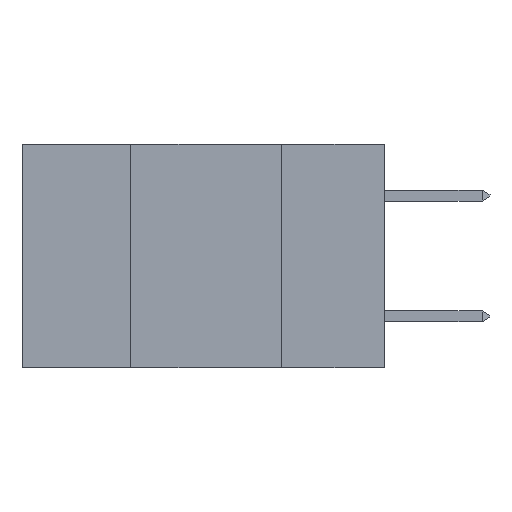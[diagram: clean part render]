
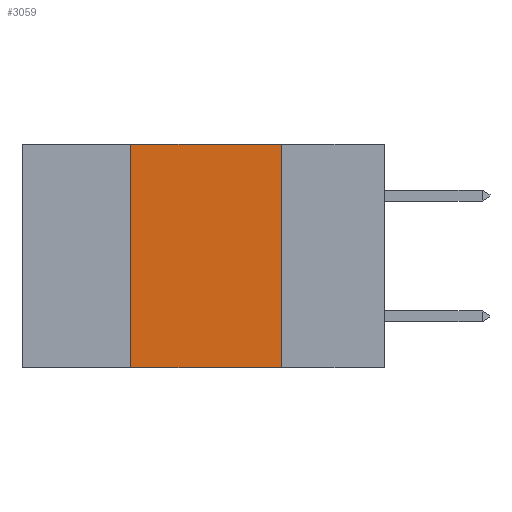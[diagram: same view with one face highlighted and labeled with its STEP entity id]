
A CAD part, left-side view. The second image highlights one B-rep face of the part: STEP entity #3059.
In plain terms, the highlighted planar face has unit normal (-1, 0, 0).
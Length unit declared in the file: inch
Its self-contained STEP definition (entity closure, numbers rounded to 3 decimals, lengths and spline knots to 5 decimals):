
#133 = VECTOR ( 'NONE', #5936, 39.37008 ) ;
#2025 = CARTESIAN_POINT ( 'NONE',  ( 0., 0.17, 0. ) ) ;
#3059 = ADVANCED_FACE ( 'NONE', ( #3275 ), #4996, .F. ) ;
#3275 = FACE_OUTER_BOUND ( 'NONE', #11206, .T. ) ;
#3481 = DIRECTION ( 'NONE',  ( 1., 0., 0. ) ) ;
#4345 = CARTESIAN_POINT ( 'NONE',  ( 0., 0.42, 0. ) ) ;
#4996 = PLANE ( 'NONE',  #13229 ) ;
#5587 = EDGE_CURVE ( 'NONE', #12993, #18678, #8573, .T. ) ;
#5814 = VERTEX_POINT ( 'NONE', #18926 ) ;
#5936 = DIRECTION ( 'NONE',  ( 0., 0., 1. ) ) ;
#6013 = ORIENTED_EDGE ( 'NONE', *, *, #13463, .F. ) ;
#7469 = ORIENTED_EDGE ( 'NONE', *, *, #20744, .F. ) ;
#7854 = ORIENTED_EDGE ( 'NONE', *, *, #13422, .F. ) ;
#8573 = LINE ( 'NONE', #15382, #11832 ) ;
#9318 = VERTEX_POINT ( 'NONE', #20121 ) ;
#9936 = CARTESIAN_POINT ( 'NONE',  ( 0., 0.6, 0. ) ) ;
#11185 = LINE ( 'NONE', #12137, #12690 ) ;
#11206 = EDGE_LOOP ( 'NONE', ( #7469, #7854, #6013, #16573 ) ) ;
#11832 = VECTOR ( 'NONE', #15319, 39.37008 ) ;
#11939 = LINE ( 'NONE', #4345, #133 ) ;
#12137 = CARTESIAN_POINT ( 'NONE',  ( 0., 0.6, 0. ) ) ;
#12690 = VECTOR ( 'NONE', #12712, 39.37008 ) ;
#12712 = DIRECTION ( 'NONE',  ( 0., -1., 0. ) ) ;
#12993 = VERTEX_POINT ( 'NONE', #19839 ) ;
#13229 = AXIS2_PLACEMENT_3D ( 'NONE', #9936, #3481, #16271 ) ;
#13422 = EDGE_CURVE ( 'NONE', #9318, #5814, #11185, .T. ) ;
#13463 = EDGE_CURVE ( 'NONE', #12993, #9318, #11939, .T. ) ;
#13984 = LINE ( 'NONE', #2025, #14480 ) ;
#14480 = VECTOR ( 'NONE', #19809, 39.37008 ) ;
#15319 = DIRECTION ( 'NONE',  ( 0., -1., 0. ) ) ;
#15382 = CARTESIAN_POINT ( 'NONE',  ( 0., 0.6, -0.37 ) ) ;
#16271 = DIRECTION ( 'NONE',  ( 0., 0., -1. ) ) ;
#16573 = ORIENTED_EDGE ( 'NONE', *, *, #5587, .T. ) ;
#18247 = CARTESIAN_POINT ( 'NONE',  ( 0., 0.17, -0.37 ) ) ;
#18678 = VERTEX_POINT ( 'NONE', #18247 ) ;
#18926 = CARTESIAN_POINT ( 'NONE',  ( 0., 0.17, 0. ) ) ;
#19809 = DIRECTION ( 'NONE',  ( 0., 0., -1. ) ) ;
#19839 = CARTESIAN_POINT ( 'NONE',  ( 0., 0.42, -0.37 ) ) ;
#20121 = CARTESIAN_POINT ( 'NONE',  ( 0., 0.42, 0. ) ) ;
#20744 = EDGE_CURVE ( 'NONE', #5814, #18678, #13984, .T. ) ;
